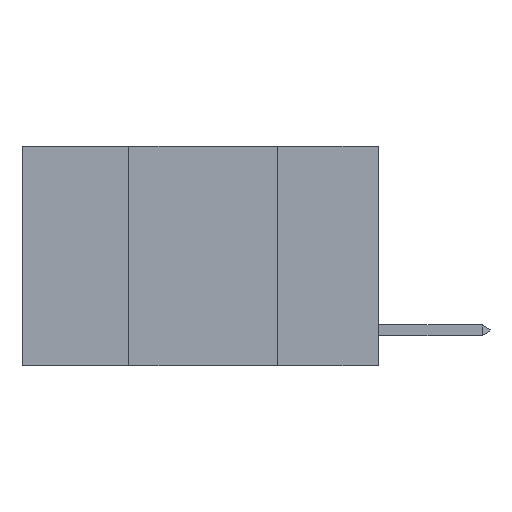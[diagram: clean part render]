
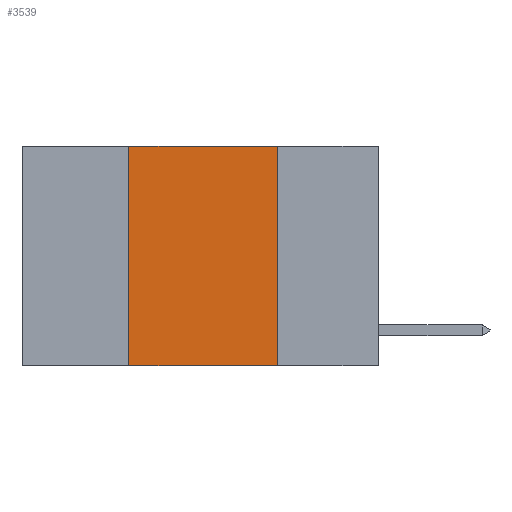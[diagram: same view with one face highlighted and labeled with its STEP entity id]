
A CAD part, left-side view. The second image highlights one B-rep face of the part: STEP entity #3539.
In plain terms, the highlighted planar face has unit normal (-1, 0, 0).
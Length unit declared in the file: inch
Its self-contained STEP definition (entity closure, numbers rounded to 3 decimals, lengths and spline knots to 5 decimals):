
#341 = ORIENTED_EDGE ( 'NONE', *, *, #2219, .T. ) ;
#352 = CARTESIAN_POINT ( 'NONE',  ( 0., 0.17, -0.37 ) ) ;
#1412 = DIRECTION ( 'NONE',  ( 0., -1., 0. ) ) ;
#1536 = FACE_OUTER_BOUND ( 'NONE', #11840, .T. ) ;
#1972 = LINE ( 'NONE', #13065, #9690 ) ;
#2106 = AXIS2_PLACEMENT_3D ( 'NONE', #5548, #11532, #9588 ) ;
#2219 = EDGE_CURVE ( 'NONE', #5263, #9812, #10454, .T. ) ;
#2594 = EDGE_CURVE ( 'NONE', #4832, #3957, #1972, .T. ) ;
#2907 = CARTESIAN_POINT ( 'NONE',  ( 0., 0.42, -0.37 ) ) ;
#3138 = VECTOR ( 'NONE', #3936, 39.37008 ) ;
#3537 = CARTESIAN_POINT ( 'NONE',  ( 0., 0.42, 0. ) ) ;
#3539 = ADVANCED_FACE ( 'NONE', ( #1536 ), #10388, .F. ) ;
#3758 = EDGE_CURVE ( 'NONE', #5263, #4832, #10245, .T. ) ;
#3936 = DIRECTION ( 'NONE',  ( 0., 0., -1. ) ) ;
#3957 = VERTEX_POINT ( 'NONE', #8242 ) ;
#3989 = DIRECTION ( 'NONE',  ( 0., -1., 0. ) ) ;
#4258 = CARTESIAN_POINT ( 'NONE',  ( 0., 0.6, -0.37 ) ) ;
#4563 = ORIENTED_EDGE ( 'NONE', *, *, #3758, .F. ) ;
#4832 = VERTEX_POINT ( 'NONE', #3537 ) ;
#5216 = DIRECTION ( 'NONE',  ( 0., 0., 1. ) ) ;
#5263 = VERTEX_POINT ( 'NONE', #2907 ) ;
#5548 = CARTESIAN_POINT ( 'NONE',  ( 0., 0.6, 0. ) ) ;
#5557 = ORIENTED_EDGE ( 'NONE', *, *, #10414, .F. ) ;
#5925 = CARTESIAN_POINT ( 'NONE',  ( 0., 0.42, 0. ) ) ;
#6700 = ORIENTED_EDGE ( 'NONE', *, *, #2594, .F. ) ;
#8242 = CARTESIAN_POINT ( 'NONE',  ( 0., 0.17, 0. ) ) ;
#8265 = VECTOR ( 'NONE', #5216, 39.37008 ) ;
#9588 = DIRECTION ( 'NONE',  ( 0., 0., -1. ) ) ;
#9690 = VECTOR ( 'NONE', #3989, 39.37008 ) ;
#9812 = VERTEX_POINT ( 'NONE', #352 ) ;
#10245 = LINE ( 'NONE', #5925, #8265 ) ;
#10388 = PLANE ( 'NONE',  #2106 ) ;
#10414 = EDGE_CURVE ( 'NONE', #3957, #9812, #11111, .T. ) ;
#10454 = LINE ( 'NONE', #4258, #10665 ) ;
#10665 = VECTOR ( 'NONE', #1412, 39.37008 ) ;
#11111 = LINE ( 'NONE', #13003, #3138 ) ;
#11532 = DIRECTION ( 'NONE',  ( 1., 0., 0. ) ) ;
#11840 = EDGE_LOOP ( 'NONE', ( #5557, #6700, #4563, #341 ) ) ;
#13003 = CARTESIAN_POINT ( 'NONE',  ( 0., 0.17, 0. ) ) ;
#13065 = CARTESIAN_POINT ( 'NONE',  ( 0., 0.6, 0. ) ) ;
